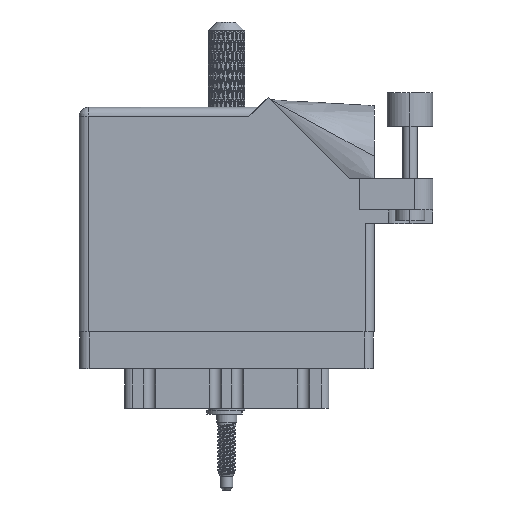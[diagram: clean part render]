
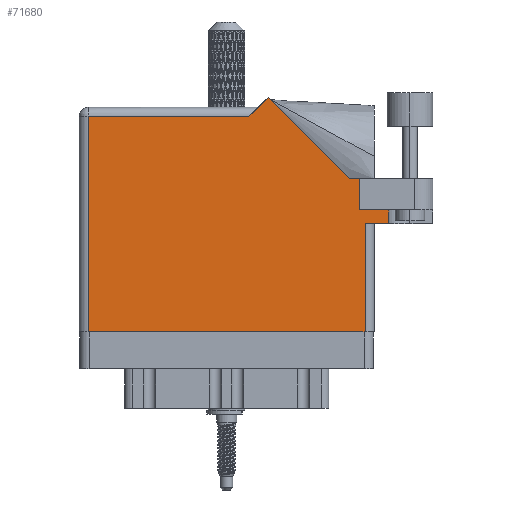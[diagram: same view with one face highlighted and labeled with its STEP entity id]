
A CAD part, front view. The second image highlights one B-rep face of the part: STEP entity #71680.
In plain terms, the highlighted face is planar.
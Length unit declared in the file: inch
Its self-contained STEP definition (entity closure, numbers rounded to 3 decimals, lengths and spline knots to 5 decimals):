
#2623 = VECTOR ( 'NONE', #54550, 39.37008 ) ;
#3153 = VECTOR ( 'NONE', #99593, 39.37008 ) ;
#3262 = VERTEX_POINT ( 'NONE', #11661 ) ;
#6749 = DIRECTION ( 'NONE',  ( 0., 0., -1. ) ) ;
#6812 = VECTOR ( 'NONE', #92100, 39.37008 ) ;
#7279 = FACE_OUTER_BOUND ( 'NONE', #103081, .T. ) ;
#8794 = CARTESIAN_POINT ( 'NONE',  ( 1.948, 0.737, 0. ) ) ;
#8833 = CARTESIAN_POINT ( 'NONE',  ( 0., 1.468, 0. ) ) ;
#9328 = VERTEX_POINT ( 'NONE', #18546 ) ;
#10251 = VERTEX_POINT ( 'NONE', #41692 ) ;
#10355 = CARTESIAN_POINT ( 'NONE',  ( 0.062, 1.468, 0. ) ) ;
#11646 = CARTESIAN_POINT ( 'NONE',  ( 1.84442, 1.044, 0. ) ) ;
#11661 = CARTESIAN_POINT ( 'NONE',  ( 1.91, 0.831, 0. ) ) ;
#12422 = VERTEX_POINT ( 'NONE', #10355 ) ;
#12566 = EDGE_CURVE ( 'NONE', #30559, #102507, #66502, .T. ) ;
#15170 = DIRECTION ( 'NONE',  ( 1., 0., 0. ) ) ;
#15297 = ORIENTED_EDGE ( 'NONE', *, *, #94252, .T. ) ;
#18184 = VERTEX_POINT ( 'NONE', #11646 ) ;
#18359 = LINE ( 'NONE', #8833, #24374 ) ;
#18546 = CARTESIAN_POINT ( 'NONE',  ( 1.155, 1.468, 0. ) ) ;
#19551 = DIRECTION ( 'NONE',  ( 0., -1., 0. ) ) ;
#19880 = ORIENTED_EDGE ( 'NONE', *, *, #46888, .F. ) ;
#21205 = LINE ( 'NONE', #22253, #2623 ) ;
#22253 = CARTESIAN_POINT ( 'NONE',  ( 0.062, 0., 0. ) ) ;
#23120 = LINE ( 'NONE', #63877, #34227 ) ;
#24374 = VECTOR ( 'NONE', #58610, 39.37008 ) ;
#26024 = VERTEX_POINT ( 'NONE', #73616 ) ;
#27913 = VECTOR ( 'NONE', #50675, 39.37008 ) ;
#30559 = VERTEX_POINT ( 'NONE', #38317 ) ;
#30726 = CARTESIAN_POINT ( 'NONE',  ( 1.91, 1.044, 0. ) ) ;
#31106 = ORIENTED_EDGE ( 'NONE', *, *, #12566, .T. ) ;
#31692 = EDGE_CURVE ( 'NONE', #78307, #30559, #23120, .T. ) ;
#32707 = PLANE ( 'NONE',  #51541 ) ;
#34227 = VECTOR ( 'NONE', #15170, 39.37008 ) ;
#35465 = LINE ( 'NONE', #66706, #3153 ) ;
#37782 = CARTESIAN_POINT ( 'NONE',  ( 1.84442, 1.044, 0. ) ) ;
#38317 = CARTESIAN_POINT ( 'NONE',  ( 1.948, 0., 0. ) ) ;
#38917 = VERTEX_POINT ( 'NONE', #30726 ) ;
#41132 = LINE ( 'NONE', #97864, #96563 ) ;
#41304 = LINE ( 'NONE', #97526, #41801 ) ;
#41692 = CARTESIAN_POINT ( 'NONE',  ( 1.28771, 1.60071, 0. ) ) ;
#41801 = VECTOR ( 'NONE', #72054, 39.37008 ) ;
#46888 = EDGE_CURVE ( 'NONE', #3262, #73766, #41304, .T. ) ;
#48016 = ORIENTED_EDGE ( 'NONE', *, *, #31692, .T. ) ;
#49726 = CARTESIAN_POINT ( 'NONE',  ( 2.1115, 1.16177, 0. ) ) ;
#50675 = DIRECTION ( 'NONE',  ( -1., 0., 0. ) ) ;
#50729 = CARTESIAN_POINT ( 'NONE',  ( 2.01, 0.737, 0. ) ) ;
#51123 = DIRECTION ( 'NONE',  ( 0., 1., 0. ) ) ;
#51541 = AXIS2_PLACEMENT_3D ( 'NONE', #94730, #6749, #96323 ) ;
#52013 = EDGE_CURVE ( 'NONE', #3262, #38917, #41132, .T. ) ;
#54550 = DIRECTION ( 'NONE',  ( 0., -1., 0. ) ) ;
#57334 = DIRECTION ( 'NONE',  ( -0.707, 0.707, 0. ) ) ;
#57557 = DIRECTION ( 'NONE',  ( 0., 1., 0. ) ) ;
#58610 = DIRECTION ( 'NONE',  ( -1., 0., 0. ) ) ;
#59308 = ORIENTED_EDGE ( 'NONE', *, *, #99793, .F. ) ;
#59341 = ORIENTED_EDGE ( 'NONE', *, *, #84791, .T. ) ;
#60509 = EDGE_CURVE ( 'NONE', #102507, #26024, #67171, .T. ) ;
#61604 = CARTESIAN_POINT ( 'NONE',  ( 2.1115, 0.831, 0. ) ) ;
#63027 = CARTESIAN_POINT ( 'NONE',  ( 1.948, 0.737, 0. ) ) ;
#63877 = CARTESIAN_POINT ( 'NONE',  ( 0., 0., 0. ) ) ;
#66502 = LINE ( 'NONE', #8794, #89161 ) ;
#66706 = CARTESIAN_POINT ( 'NONE',  ( 1.217, 1.53, 0. ) ) ;
#67171 = LINE ( 'NONE', #50729, #6812 ) ;
#68303 = ORIENTED_EDGE ( 'NONE', *, *, #52013, .T. ) ;
#69238 = ORIENTED_EDGE ( 'NONE', *, *, #96065, .T. ) ;
#71680 = ADVANCED_FACE ( 'NONE', ( #7279 ), #32707, .F. ) ;
#72054 = DIRECTION ( 'NONE',  ( 1., 0., 0. ) ) ;
#73489 = LINE ( 'NONE', #97917, #27913 ) ;
#73616 = CARTESIAN_POINT ( 'NONE',  ( 2.1115, 0.737, 0. ) ) ;
#73766 = VERTEX_POINT ( 'NONE', #61604 ) ;
#76194 = LINE ( 'NONE', #49726, #102434 ) ;
#78307 = VERTEX_POINT ( 'NONE', #81575 ) ;
#80664 = LINE ( 'NONE', #37782, #104125 ) ;
#81575 = CARTESIAN_POINT ( 'NONE',  ( 0.062, 0., 0. ) ) ;
#84791 = EDGE_CURVE ( 'NONE', #10251, #9328, #35465, .T. ) ;
#89161 = VECTOR ( 'NONE', #51123, 39.37008 ) ;
#89507 = ORIENTED_EDGE ( 'NONE', *, *, #60509, .T. ) ;
#91930 = ORIENTED_EDGE ( 'NONE', *, *, #100746, .T. ) ;
#92100 = DIRECTION ( 'NONE',  ( 1., 0., 0. ) ) ;
#92697 = ORIENTED_EDGE ( 'NONE', *, *, #101455, .T. ) ;
#94252 = EDGE_CURVE ( 'NONE', #9328, #12422, #18359, .T. ) ;
#94730 = CARTESIAN_POINT ( 'NONE',  ( 0., 1.53, 0. ) ) ;
#96065 = EDGE_CURVE ( 'NONE', #38917, #18184, #73489, .T. ) ;
#96323 = DIRECTION ( 'NONE',  ( -1., 0., 0. ) ) ;
#96563 = VECTOR ( 'NONE', #57557, 39.37008 ) ;
#97526 = CARTESIAN_POINT ( 'NONE',  ( 1.91, 0.831, 0. ) ) ;
#97864 = CARTESIAN_POINT ( 'NONE',  ( 1.91, 0.831, 0. ) ) ;
#97917 = CARTESIAN_POINT ( 'NONE',  ( 2.41, 1.044, 0. ) ) ;
#99593 = DIRECTION ( 'NONE',  ( -0.707, -0.707, 0. ) ) ;
#99793 = EDGE_CURVE ( 'NONE', #73766, #26024, #76194, .T. ) ;
#100746 = EDGE_CURVE ( 'NONE', #18184, #10251, #80664, .T. ) ;
#101455 = EDGE_CURVE ( 'NONE', #12422, #78307, #21205, .T. ) ;
#102434 = VECTOR ( 'NONE', #19551, 39.37008 ) ;
#102507 = VERTEX_POINT ( 'NONE', #63027 ) ;
#103081 = EDGE_LOOP ( 'NONE', ( #48016, #31106, #89507, #59308, #19880, #68303, #69238, #91930, #59341, #15297, #92697 ) ) ;
#104125 = VECTOR ( 'NONE', #57334, 39.37008 ) ;
